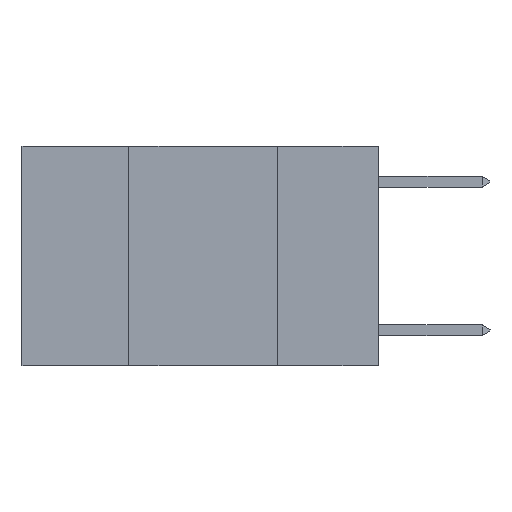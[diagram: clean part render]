
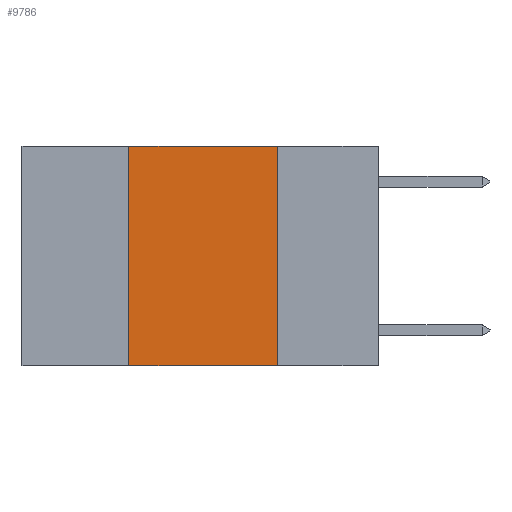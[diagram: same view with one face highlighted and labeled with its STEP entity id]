
A CAD part, left-side view. The second image highlights one B-rep face of the part: STEP entity #9786.
In plain terms, the highlighted planar face has unit normal (-1, 0, 0).
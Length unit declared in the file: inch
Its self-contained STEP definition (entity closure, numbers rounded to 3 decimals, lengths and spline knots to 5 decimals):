
#333 = CARTESIAN_POINT ( 'NONE',  ( 0., 0.6, 0. ) ) ;
#464 = ORIENTED_EDGE ( 'NONE', *, *, #2637, .T. ) ;
#563 = EDGE_CURVE ( 'NONE', #3961, #1021, #580, .T. ) ;
#580 = LINE ( 'NONE', #7436, #2516 ) ;
#586 = EDGE_CURVE ( 'NONE', #5282, #3961, #4316, .T. ) ;
#714 = CARTESIAN_POINT ( 'NONE',  ( 0., 0.42, 0. ) ) ;
#1021 = VERTEX_POINT ( 'NONE', #1156 ) ;
#1156 = CARTESIAN_POINT ( 'NONE',  ( 0., 0.17, -0.37 ) ) ;
#1351 = VECTOR ( 'NONE', #2980, 39.37008 ) ;
#1981 = CARTESIAN_POINT ( 'NONE',  ( 0., 0.42, -0.37 ) ) ;
#2165 = ORIENTED_EDGE ( 'NONE', *, *, #563, .F. ) ;
#2252 = VECTOR ( 'NONE', #8409, 39.37008 ) ;
#2256 = DIRECTION ( 'NONE',  ( 0., 0., -1. ) ) ;
#2275 = VECTOR ( 'NONE', #3311, 39.37008 ) ;
#2417 = CARTESIAN_POINT ( 'NONE',  ( 0., 0.42, 0. ) ) ;
#2488 = LINE ( 'NONE', #714, #2252 ) ;
#2490 = EDGE_CURVE ( 'NONE', #7570, #5282, #2488, .T. ) ;
#2516 = VECTOR ( 'NONE', #2256, 39.37008 ) ;
#2525 = PLANE ( 'NONE',  #8140 ) ;
#2637 = EDGE_CURVE ( 'NONE', #7570, #1021, #7618, .T. ) ;
#2980 = DIRECTION ( 'NONE',  ( 0., -1., 0. ) ) ;
#3059 = CARTESIAN_POINT ( 'NONE',  ( 0., 0.17, 0. ) ) ;
#3283 = DIRECTION ( 'NONE',  ( 0., 0., -1. ) ) ;
#3311 = DIRECTION ( 'NONE',  ( 0., -1., 0. ) ) ;
#3543 = EDGE_LOOP ( 'NONE', ( #2165, #9477, #4199, #464 ) ) ;
#3961 = VERTEX_POINT ( 'NONE', #3059 ) ;
#4199 = ORIENTED_EDGE ( 'NONE', *, *, #2490, .F. ) ;
#4316 = LINE ( 'NONE', #8789, #2275 ) ;
#5282 = VERTEX_POINT ( 'NONE', #2417 ) ;
#5481 = FACE_OUTER_BOUND ( 'NONE', #3543, .T. ) ;
#7436 = CARTESIAN_POINT ( 'NONE',  ( 0., 0.17, 0. ) ) ;
#7570 = VERTEX_POINT ( 'NONE', #1981 ) ;
#7618 = LINE ( 'NONE', #9249, #1351 ) ;
#8064 = DIRECTION ( 'NONE',  ( 1., 0., 0. ) ) ;
#8140 = AXIS2_PLACEMENT_3D ( 'NONE', #333, #8064, #3283 ) ;
#8409 = DIRECTION ( 'NONE',  ( 0., 0., 1. ) ) ;
#8789 = CARTESIAN_POINT ( 'NONE',  ( 0., 0.6, 0. ) ) ;
#9249 = CARTESIAN_POINT ( 'NONE',  ( 0., 0.6, -0.37 ) ) ;
#9477 = ORIENTED_EDGE ( 'NONE', *, *, #586, .F. ) ;
#9786 = ADVANCED_FACE ( 'NONE', ( #5481 ), #2525, .F. ) ;
